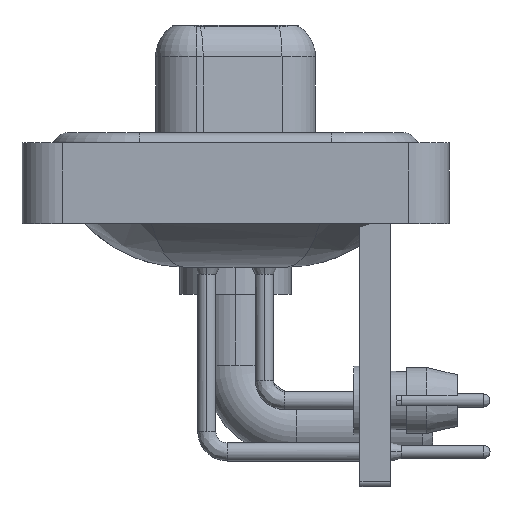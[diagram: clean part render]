
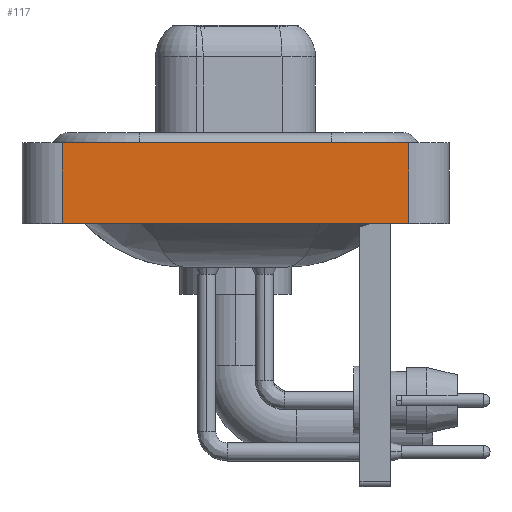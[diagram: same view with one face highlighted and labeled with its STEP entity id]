
A CAD part, left-side view. The second image highlights one B-rep face of the part: STEP entity #117.
In plain terms, the highlighted planar face has unit normal (-1, 0, 0).
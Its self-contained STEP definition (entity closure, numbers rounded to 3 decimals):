
#117 = ADVANCED_FACE ( 'NONE', ( #18265 ), #11668, .T. ) ;
#261 = CARTESIAN_POINT ( 'NONE',  ( -7.25, -8.55, 0.4 ) ) ;
#554 = DIRECTION ( 'NONE',  ( 0., -1., 0. ) ) ;
#606 = VECTOR ( 'NONE', #6762, 1000. ) ;
#2654 = VECTOR ( 'NONE', #10750, 1000. ) ;
#2764 = DIRECTION ( 'NONE',  ( 0., 0., 1. ) ) ;
#4615 = CARTESIAN_POINT ( 'NONE',  ( -7.25, 8.55, 0.4 ) ) ;
#5352 = EDGE_CURVE ( 'NONE', #11250, #19600, #13228, .T. ) ;
#5459 = CARTESIAN_POINT ( 'NONE',  ( -7.25, -8.55, -3.6 ) ) ;
#6762 = DIRECTION ( 'NONE',  ( 0., 0., 1. ) ) ;
#6832 = VERTEX_POINT ( 'NONE', #17186 ) ;
#7333 = CARTESIAN_POINT ( 'NONE',  ( -7.25, -8.55, 0.4 ) ) ;
#8944 = EDGE_LOOP ( 'NONE', ( #15349, #15922, #14597, #12864 ) ) ;
#10101 = CARTESIAN_POINT ( 'NONE',  ( -7.25, -8.55, -3.6 ) ) ;
#10750 = DIRECTION ( 'NONE',  ( 0., -1., 0. ) ) ;
#11052 = LINE ( 'NONE', #7333, #17495 ) ;
#11250 = VERTEX_POINT ( 'NONE', #5459 ) ;
#11668 = PLANE ( 'NONE',  #16612 ) ;
#12864 = ORIENTED_EDGE ( 'NONE', *, *, #17912, .T. ) ;
#13228 = LINE ( 'NONE', #18782, #606 ) ;
#13914 = CARTESIAN_POINT ( 'NONE',  ( -7.25, 8.55, -3.6 ) ) ;
#14597 = ORIENTED_EDGE ( 'NONE', *, *, #15425, .F. ) ;
#15349 = ORIENTED_EDGE ( 'NONE', *, *, #5352, .T. ) ;
#15425 = EDGE_CURVE ( 'NONE', #6832, #16791, #17546, .T. ) ;
#15922 = ORIENTED_EDGE ( 'NONE', *, *, #18514, .F. ) ;
#16612 = AXIS2_PLACEMENT_3D ( 'NONE', #10101, #18587, #2764 ) ;
#16791 = VERTEX_POINT ( 'NONE', #4615 ) ;
#17186 = CARTESIAN_POINT ( 'NONE',  ( -7.25, 8.55, -3.6 ) ) ;
#17495 = VECTOR ( 'NONE', #554, 1000. ) ;
#17546 = LINE ( 'NONE', #13914, #18642 ) ;
#17912 = EDGE_CURVE ( 'NONE', #6832, #11250, #21086, .T. ) ;
#18265 = FACE_OUTER_BOUND ( 'NONE', #8944, .T. ) ;
#18514 = EDGE_CURVE ( 'NONE', #16791, #19600, #11052, .T. ) ;
#18587 = DIRECTION ( 'NONE',  ( -1., 0., 0. ) ) ;
#18642 = VECTOR ( 'NONE', #21700, 1000. ) ;
#18782 = CARTESIAN_POINT ( 'NONE',  ( -7.25, -8.55, -3.6 ) ) ;
#18911 = CARTESIAN_POINT ( 'NONE',  ( -7.25, -8.55, -3.6 ) ) ;
#19600 = VERTEX_POINT ( 'NONE', #261 ) ;
#21086 = LINE ( 'NONE', #18911, #2654 ) ;
#21700 = DIRECTION ( 'NONE',  ( 0., 0., 1. ) ) ;
